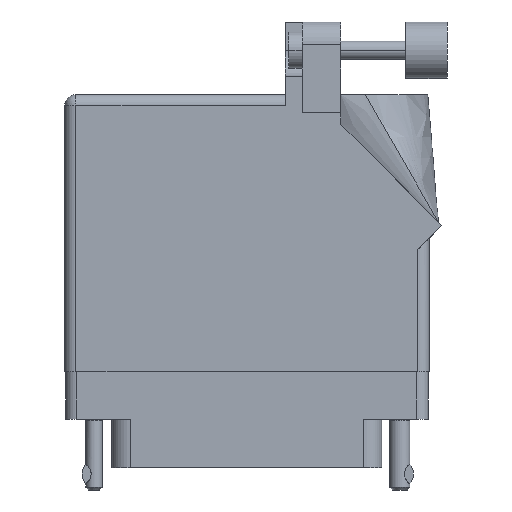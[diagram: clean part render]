
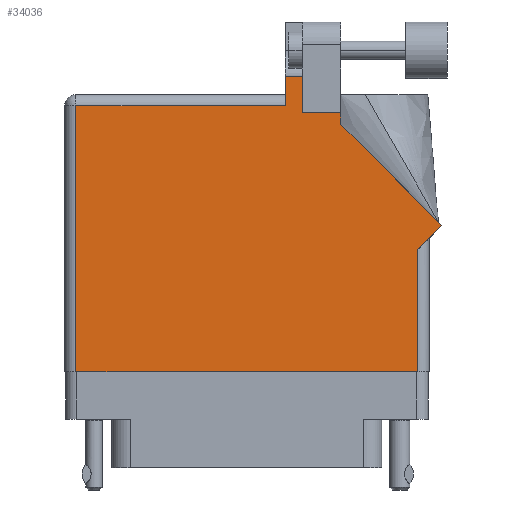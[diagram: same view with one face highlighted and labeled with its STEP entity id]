
A CAD part, front view. The second image highlights one B-rep face of the part: STEP entity #34036.
In plain terms, the highlighted face is planar.
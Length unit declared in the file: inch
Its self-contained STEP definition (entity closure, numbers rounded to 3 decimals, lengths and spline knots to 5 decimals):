
#685 = LINE ( 'NONE', #33401, #38452 ) ;
#728 = CARTESIAN_POINT ( 'NONE',  ( 0., 0., 0. ) ) ;
#1069 = VECTOR ( 'NONE', #28305, 39.37008 ) ;
#1612 = LINE ( 'NONE', #728, #1069 ) ;
#1998 = ORIENTED_EDGE ( 'NONE', *, *, #34970, .T. ) ;
#2143 = VERTEX_POINT ( 'NONE', #38366 ) ;
#2531 = VERTEX_POINT ( 'NONE', #22907 ) ;
#2902 = DIRECTION ( 'NONE',  ( 0., 1., 0. ) ) ;
#3052 = VERTEX_POINT ( 'NONE', #8788 ) ;
#3647 = DIRECTION ( 'NONE',  ( 0., 1., 0. ) ) ;
#3884 = LINE ( 'NONE', #33175, #5004 ) ;
#4770 = LINE ( 'NONE', #22988, #23129 ) ;
#4910 = FACE_OUTER_BOUND ( 'NONE', #33219, .T. ) ;
#5004 = VECTOR ( 'NONE', #26267, 39.37008 ) ;
#5820 = ORIENTED_EDGE ( 'NONE', *, *, #8843, .T. ) ;
#6244 = LINE ( 'NONE', #39877, #42986 ) ;
#7320 = CARTESIAN_POINT ( 'NONE',  ( 2.08071, 0.80771, 0. ) ) ;
#7721 = VERTEX_POINT ( 'NONE', #32242 ) ;
#7830 = LINE ( 'NONE', #19927, #38591 ) ;
#8788 = CARTESIAN_POINT ( 'NONE',  ( 1.217, 1.468, 0. ) ) ;
#8843 = EDGE_CURVE ( 'NONE', #2531, #15451, #39428, .T. ) ;
#9010 = PLANE ( 'NONE',  #36460 ) ;
#10896 = CARTESIAN_POINT ( 'NONE',  ( 1.311, 1.43, 0. ) ) ;
#11138 = EDGE_CURVE ( 'NONE', #13311, #29498, #39302, .T. ) ;
#11739 = ORIENTED_EDGE ( 'NONE', *, *, #35729, .T. ) ;
#12903 = EDGE_CURVE ( 'NONE', #14847, #28157, #35982, .T. ) ;
#13030 = ORIENTED_EDGE ( 'NONE', *, *, #12903, .T. ) ;
#13311 = VERTEX_POINT ( 'NONE', #43200 ) ;
#13480 = CARTESIAN_POINT ( 'NONE',  ( 0., 1.53, 0. ) ) ;
#13588 = EDGE_CURVE ( 'NONE', #7721, #38168, #7830, .T. ) ;
#14847 = VERTEX_POINT ( 'NONE', #15630 ) ;
#15285 = CARTESIAN_POINT ( 'NONE',  ( 1.217, 1.6315, 0. ) ) ;
#15451 = VERTEX_POINT ( 'NONE', #22102 ) ;
#15550 = DIRECTION ( 'NONE',  ( 0., 0., -1. ) ) ;
#15630 = CARTESIAN_POINT ( 'NONE',  ( 1.948, 0., 0. ) ) ;
#16829 = ORIENTED_EDGE ( 'NONE', *, *, #27962, .T. ) ;
#19246 = LINE ( 'NONE', #20361, #38064 ) ;
#19927 = CARTESIAN_POINT ( 'NONE',  ( 1.64177, 1.6315, 0. ) ) ;
#20361 = CARTESIAN_POINT ( 'NONE',  ( 1.217, 1.53, 0. ) ) ;
#20959 = DIRECTION ( 'NONE',  ( -1., 0., 0. ) ) ;
#21068 = DIRECTION ( 'NONE',  ( -0.707, 0.707, 0. ) ) ;
#22102 = CARTESIAN_POINT ( 'NONE',  ( 1.311, 1.43, 0. ) ) ;
#22907 = CARTESIAN_POINT ( 'NONE',  ( 1.524, 1.43, 0. ) ) ;
#22931 = DIRECTION ( 'NONE',  ( 0., -1., 0. ) ) ;
#22988 = CARTESIAN_POINT ( 'NONE',  ( 0.062, 0., 0. ) ) ;
#23129 = VECTOR ( 'NONE', #29610, 39.37008 ) ;
#23856 = VERTEX_POINT ( 'NONE', #32056 ) ;
#25982 = DIRECTION ( 'NONE',  ( -1., 0., 0. ) ) ;
#26267 = DIRECTION ( 'NONE',  ( 0., 1., 0. ) ) ;
#26497 = DIRECTION ( 'NONE',  ( 0.707, 0.707, 0. ) ) ;
#27188 = EDGE_CURVE ( 'NONE', #15451, #7721, #30037, .T. ) ;
#27962 = EDGE_CURVE ( 'NONE', #3052, #2143, #6244, .T. ) ;
#28157 = VERTEX_POINT ( 'NONE', #33936 ) ;
#28305 = DIRECTION ( 'NONE',  ( 1., 0., 0. ) ) ;
#28541 = ORIENTED_EDGE ( 'NONE', *, *, #13588, .T. ) ;
#28911 = ORIENTED_EDGE ( 'NONE', *, *, #11138, .T. ) ;
#29498 = VERTEX_POINT ( 'NONE', #37324 ) ;
#29610 = DIRECTION ( 'NONE',  ( 0., -1., 0. ) ) ;
#30037 = LINE ( 'NONE', #10896, #36576 ) ;
#30730 = EDGE_CURVE ( 'NONE', #28157, #13311, #685, .T. ) ;
#31069 = VECTOR ( 'NONE', #2902, 39.37008 ) ;
#31946 = ORIENTED_EDGE ( 'NONE', *, *, #42870, .T. ) ;
#32056 = CARTESIAN_POINT ( 'NONE',  ( 0.062, 0., 0. ) ) ;
#32242 = CARTESIAN_POINT ( 'NONE',  ( 1.311, 1.6315, 0. ) ) ;
#33175 = CARTESIAN_POINT ( 'NONE',  ( 1.524, 1.36442, 0. ) ) ;
#33219 = EDGE_LOOP ( 'NONE', ( #35498, #28541, #31946, #16829, #11739, #1998, #13030, #34893, #28911, #38743, #5820 ) ) ;
#33401 = CARTESIAN_POINT ( 'NONE',  ( 2.01, 0.737, 0. ) ) ;
#33936 = CARTESIAN_POINT ( 'NONE',  ( 1.948, 0.675, 0. ) ) ;
#34036 = ADVANCED_FACE ( 'NONE', ( #4910 ), #9010, .F. ) ;
#34546 = VECTOR ( 'NONE', #39886, 39.37008 ) ;
#34893 = ORIENTED_EDGE ( 'NONE', *, *, #30730, .T. ) ;
#34970 = EDGE_CURVE ( 'NONE', #23856, #14847, #1612, .T. ) ;
#35498 = ORIENTED_EDGE ( 'NONE', *, *, #27188, .T. ) ;
#35729 = EDGE_CURVE ( 'NONE', #2143, #23856, #4770, .T. ) ;
#35982 = LINE ( 'NONE', #44408, #31069 ) ;
#36460 = AXIS2_PLACEMENT_3D ( 'NONE', #13480, #15550, #44189 ) ;
#36576 = VECTOR ( 'NONE', #3647, 39.37008 ) ;
#37125 = VECTOR ( 'NONE', #21068, 39.37008 ) ;
#37324 = CARTESIAN_POINT ( 'NONE',  ( 1.524, 1.36442, 0. ) ) ;
#38064 = VECTOR ( 'NONE', #22931, 39.37008 ) ;
#38168 = VERTEX_POINT ( 'NONE', #15285 ) ;
#38366 = CARTESIAN_POINT ( 'NONE',  ( 0.062, 1.468, 0. ) ) ;
#38452 = VECTOR ( 'NONE', #26497, 39.37008 ) ;
#38591 = VECTOR ( 'NONE', #20959, 39.37008 ) ;
#38743 = ORIENTED_EDGE ( 'NONE', *, *, #40480, .T. ) ;
#39302 = LINE ( 'NONE', #7320, #37125 ) ;
#39428 = LINE ( 'NONE', #40175, #34546 ) ;
#39877 = CARTESIAN_POINT ( 'NONE',  ( 0., 1.468, 0. ) ) ;
#39886 = DIRECTION ( 'NONE',  ( -1., 0., 0. ) ) ;
#40175 = CARTESIAN_POINT ( 'NONE',  ( 1.524, 1.43, 0. ) ) ;
#40480 = EDGE_CURVE ( 'NONE', #29498, #2531, #3884, .T. ) ;
#42870 = EDGE_CURVE ( 'NONE', #38168, #3052, #19246, .T. ) ;
#42986 = VECTOR ( 'NONE', #25982, 39.37008 ) ;
#43200 = CARTESIAN_POINT ( 'NONE',  ( 2.08071, 0.80771, 0. ) ) ;
#44189 = DIRECTION ( 'NONE',  ( -1., 0., 0. ) ) ;
#44408 = CARTESIAN_POINT ( 'NONE',  ( 1.948, 0.737, 0. ) ) ;
